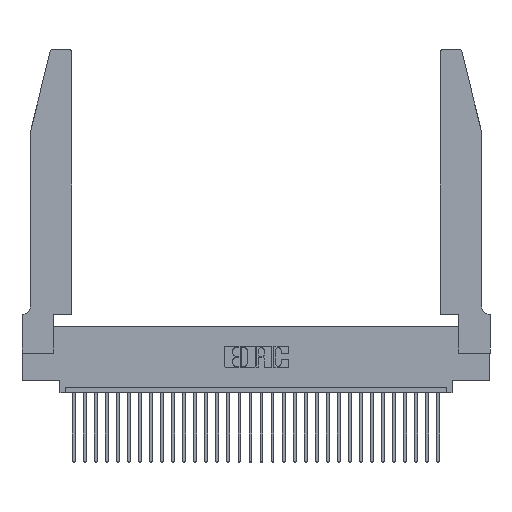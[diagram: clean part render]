
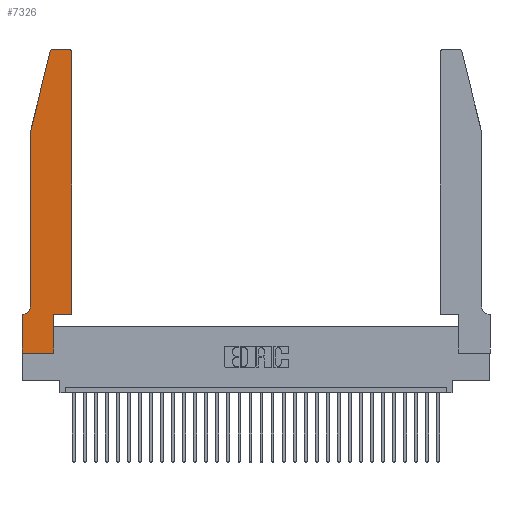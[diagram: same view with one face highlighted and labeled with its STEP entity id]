
A CAD part, top view. The second image highlights one B-rep face of the part: STEP entity #7326.
In plain terms, the highlighted planar face has unit normal (0, 0, 1).
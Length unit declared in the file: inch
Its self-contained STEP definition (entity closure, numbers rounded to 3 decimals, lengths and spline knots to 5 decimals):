
#334 = VECTOR ( 'NONE', #18177, 39.37008 ) ;
#467 = CARTESIAN_POINT ( 'NONE',  ( 0.0755, 0.35, 0.37 ) ) ;
#2016 = CARTESIAN_POINT ( 'NONE',  ( 0.0755, 2., 0.37 ) ) ;
#2582 = PLANE ( 'NONE',  #11991 ) ;
#2691 = DIRECTION ( 'NONE',  ( -0.239, -0.971, 0. ) ) ;
#3159 = AXIS2_PLACEMENT_3D ( 'NONE', #4258, #6676, #13655 ) ;
#3347 = DIRECTION ( 'NONE',  ( -1., 0., 0. ) ) ;
#3614 = DIRECTION ( 'NONE',  ( 1., 0., 0. ) ) ;
#3631 = ORIENTED_EDGE ( 'NONE', *, *, #8871, .T. ) ;
#4120 = ORIENTED_EDGE ( 'NONE', *, *, #10845, .T. ) ;
#4258 = CARTESIAN_POINT ( 'NONE',  ( 0.0055, 0.42, 0.37 ) ) ;
#4944 = EDGE_CURVE ( 'NONE', #10950, #27281, #12985, .T. ) ;
#5267 = DIRECTION ( 'NONE',  ( 0., 0., 1. ) ) ;
#5356 = CARTESIAN_POINT ( 'NONE',  ( 0.284, 2.75, 0.37 ) ) ;
#5537 = ORIENTED_EDGE ( 'NONE', *, *, #8664, .T. ) ;
#5882 = DIRECTION ( 'NONE',  ( 0., 0., 1. ) ) ;
#6001 = CARTESIAN_POINT ( 'NONE',  ( 0.0755, 0.42, 0.37 ) ) ;
#6676 = DIRECTION ( 'NONE',  ( 0., 0., -1. ) ) ;
#6767 = ORIENTED_EDGE ( 'NONE', *, *, #8416, .T. ) ;
#7326 = ADVANCED_FACE ( 'NONE', ( #30831 ), #2582, .T. ) ;
#7519 = ORIENTED_EDGE ( 'NONE', *, *, #4944, .T. ) ;
#7670 = LINE ( 'NONE', #26160, #30932 ) ;
#7925 = EDGE_LOOP ( 'NONE', ( #19583, #19135, #3631, #4120, #17276, #17804, #22328, #7519, #6767, #5537, #27268, #27560 ) ) ;
#8112 = LINE ( 'NONE', #20669, #13812 ) ;
#8304 = DIRECTION ( 'NONE',  ( 1., 0., 0. ) ) ;
#8305 = CARTESIAN_POINT ( 'NONE',  ( 0.2605, 2.75, 0.37 ) ) ;
#8416 = EDGE_CURVE ( 'NONE', #27281, #19775, #7670, .T. ) ;
#8510 = VECTOR ( 'NONE', #2691, 39.37008 ) ;
#8664 = EDGE_CURVE ( 'NONE', #19775, #16135, #8112, .T. ) ;
#8871 = EDGE_CURVE ( 'NONE', #27264, #16396, #14976, .T. ) ;
#9413 = CARTESIAN_POINT ( 'NONE',  ( 0., 0.35, 0.37 ) ) ;
#9458 = VERTEX_POINT ( 'NONE', #5356 ) ;
#9515 = VERTEX_POINT ( 'NONE', #6001 ) ;
#9860 = EDGE_CURVE ( 'NONE', #23025, #17433, #19874, .T. ) ;
#10109 = DIRECTION ( 'NONE',  ( 1., 0., 0. ) ) ;
#10162 = VECTOR ( 'NONE', #26466, 39.37008 ) ;
#10845 = EDGE_CURVE ( 'NONE', #16396, #9515, #30928, .T. ) ;
#10950 = VERTEX_POINT ( 'NONE', #12271 ) ;
#11991 = AXIS2_PLACEMENT_3D ( 'NONE', #29209, #29527, #29104 ) ;
#12271 = CARTESIAN_POINT ( 'NONE',  ( 0., 0., 0.37 ) ) ;
#12401 = EDGE_CURVE ( 'NONE', #16135, #23025, #20851, .T. ) ;
#12564 = VECTOR ( 'NONE', #21385, 39.37008 ) ;
#12635 = CARTESIAN_POINT ( 'NONE',  ( 0.0755, 2., 0.37 ) ) ;
#12985 = LINE ( 'NONE', #13104, #24078 ) ;
#13096 = CARTESIAN_POINT ( 'NONE',  ( 0.0755, 2., 0.37 ) ) ;
#13104 = CARTESIAN_POINT ( 'NONE',  ( 0., 0., 0.37 ) ) ;
#13287 = DIRECTION ( 'NONE',  ( 1., 0., 0. ) ) ;
#13565 = EDGE_CURVE ( 'NONE', #9458, #27264, #23834, .T. ) ;
#13655 = DIRECTION ( 'NONE',  ( -1., 0., 0. ) ) ;
#13812 = VECTOR ( 'NONE', #13287, 39.37008 ) ;
#14608 = VERTEX_POINT ( 'NONE', #9413 ) ;
#14976 = LINE ( 'NONE', #12635, #8510 ) ;
#15119 = CARTESIAN_POINT ( 'NONE',  ( 0.25487, 2.72718, 0.37 ) ) ;
#15191 = CARTESIAN_POINT ( 'NONE',  ( 0.0055, 0.35, 0.37 ) ) ;
#15860 = VECTOR ( 'NONE', #29506, 39.37008 ) ;
#16135 = VERTEX_POINT ( 'NONE', #27000 ) ;
#16396 = VERTEX_POINT ( 'NONE', #13096 ) ;
#16805 = AXIS2_PLACEMENT_3D ( 'NONE', #29751, #5267, #10109 ) ;
#17276 = ORIENTED_EDGE ( 'NONE', *, *, #29830, .T. ) ;
#17433 = VERTEX_POINT ( 'NONE', #21005 ) ;
#17804 = ORIENTED_EDGE ( 'NONE', *, *, #20641, .T. ) ;
#18177 = DIRECTION ( 'NONE',  ( -1., 0., 0. ) ) ;
#18318 = CARTESIAN_POINT ( 'NONE',  ( 0.2865, 0.35, 0.37 ) ) ;
#18540 = LINE ( 'NONE', #24236, #10162 ) ;
#19135 = ORIENTED_EDGE ( 'NONE', *, *, #13565, .T. ) ;
#19583 = ORIENTED_EDGE ( 'NONE', *, *, #22159, .T. ) ;
#19775 = VERTEX_POINT ( 'NONE', #18318 ) ;
#19874 = CIRCLE ( 'NONE', #27353, 0.03 ) ;
#20462 = EDGE_CURVE ( 'NONE', #14608, #10950, #18540, .T. ) ;
#20641 = EDGE_CURVE ( 'NONE', #25962, #14608, #26942, .T. ) ;
#20669 = CARTESIAN_POINT ( 'NONE',  ( 0.4505, 0.35, 0.37 ) ) ;
#20851 = LINE ( 'NONE', #22340, #15860 ) ;
#21005 = CARTESIAN_POINT ( 'NONE',  ( 0.4205, 2.75, 0.37 ) ) ;
#21385 = DIRECTION ( 'NONE',  ( 0., -1., 0. ) ) ;
#22159 = EDGE_CURVE ( 'NONE', #17433, #9458, #26193, .T. ) ;
#22328 = ORIENTED_EDGE ( 'NONE', *, *, #20462, .T. ) ;
#22340 = CARTESIAN_POINT ( 'NONE',  ( 0.4505, 0.35, 0.37 ) ) ;
#23025 = VERTEX_POINT ( 'NONE', #23260 ) ;
#23260 = CARTESIAN_POINT ( 'NONE',  ( 0.4505, 2.72, 0.37 ) ) ;
#23834 = CIRCLE ( 'NONE', #16805, 0.03 ) ;
#24078 = VECTOR ( 'NONE', #3614, 39.37008 ) ;
#24236 = CARTESIAN_POINT ( 'NONE',  ( 0., 0., 0.37 ) ) ;
#24637 = VECTOR ( 'NONE', #3347, 39.37008 ) ;
#25962 = VERTEX_POINT ( 'NONE', #15191 ) ;
#26160 = CARTESIAN_POINT ( 'NONE',  ( 0.2865, 0.35, 0.37 ) ) ;
#26193 = LINE ( 'NONE', #8305, #334 ) ;
#26428 = CIRCLE ( 'NONE', #3159, 0.07 ) ;
#26466 = DIRECTION ( 'NONE',  ( 0., -1., 0. ) ) ;
#26942 = LINE ( 'NONE', #467, #24637 ) ;
#27000 = CARTESIAN_POINT ( 'NONE',  ( 0.4505, 0.35, 0.37 ) ) ;
#27264 = VERTEX_POINT ( 'NONE', #15119 ) ;
#27268 = ORIENTED_EDGE ( 'NONE', *, *, #12401, .T. ) ;
#27281 = VERTEX_POINT ( 'NONE', #29989 ) ;
#27353 = AXIS2_PLACEMENT_3D ( 'NONE', #30279, #5882, #8304 ) ;
#27560 = ORIENTED_EDGE ( 'NONE', *, *, #9860, .T. ) ;
#28658 = DIRECTION ( 'NONE',  ( 0., 1., 0. ) ) ;
#29104 = DIRECTION ( 'NONE',  ( 1., 0., 0. ) ) ;
#29209 = CARTESIAN_POINT ( 'NONE',  ( 0., 0.35, 0.37 ) ) ;
#29506 = DIRECTION ( 'NONE',  ( 0., 1., 0. ) ) ;
#29527 = DIRECTION ( 'NONE',  ( 0., 0., 1. ) ) ;
#29751 = CARTESIAN_POINT ( 'NONE',  ( 0.284, 2.72, 0.37 ) ) ;
#29830 = EDGE_CURVE ( 'NONE', #9515, #25962, #26428, .T. ) ;
#29989 = CARTESIAN_POINT ( 'NONE',  ( 0.2865, 0., 0.37 ) ) ;
#30279 = CARTESIAN_POINT ( 'NONE',  ( 0.4205, 2.72, 0.37 ) ) ;
#30831 = FACE_OUTER_BOUND ( 'NONE', #7925, .T. ) ;
#30928 = LINE ( 'NONE', #2016, #12564 ) ;
#30932 = VECTOR ( 'NONE', #28658, 39.37008 ) ;
